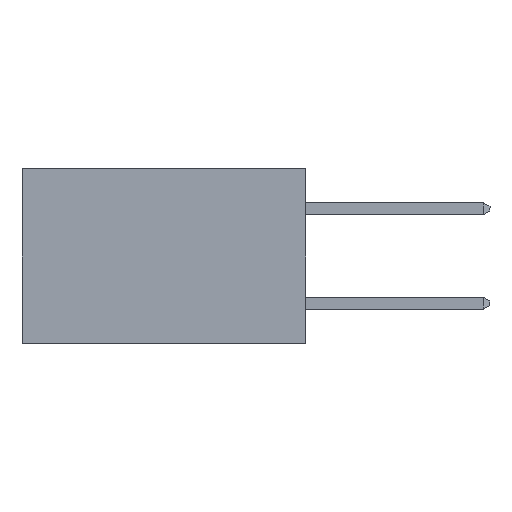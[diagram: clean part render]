
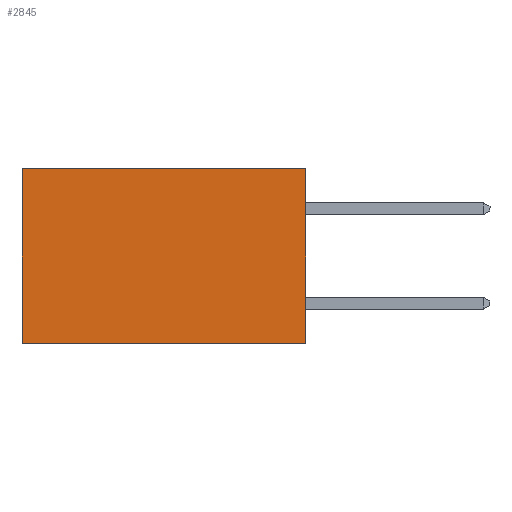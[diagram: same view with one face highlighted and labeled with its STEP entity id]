
A CAD part, left-side view. The second image highlights one B-rep face of the part: STEP entity #2845.
In plain terms, the highlighted planar face has unit normal (-1, 0, 0).
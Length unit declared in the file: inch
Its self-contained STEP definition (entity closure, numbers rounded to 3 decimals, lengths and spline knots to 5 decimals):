
#236 = EDGE_CURVE ( 'NONE', #4190, #8063, #8089, .T. ) ;
#643 = ORIENTED_EDGE ( 'NONE', *, *, #4900, .F. ) ;
#648 = VECTOR ( 'NONE', #2766, 39.37008 ) ;
#804 = VECTOR ( 'NONE', #7829, 39.37008 ) ;
#814 = CARTESIAN_POINT ( 'NONE',  ( 0.2615, 0.6, -0.37 ) ) ;
#836 = LINE ( 'NONE', #5321, #648 ) ;
#911 = LINE ( 'NONE', #2721, #804 ) ;
#1516 = FACE_OUTER_BOUND ( 'NONE', #3826, .T. ) ;
#1579 = AXIS2_PLACEMENT_3D ( 'NONE', #5293, #4053, #4133 ) ;
#1909 = VECTOR ( 'NONE', #5614, 39.37008 ) ;
#2027 = ORIENTED_EDGE ( 'NONE', *, *, #5653, .F. ) ;
#2721 = CARTESIAN_POINT ( 'NONE',  ( 0.2615, 0., -0.37 ) ) ;
#2766 = DIRECTION ( 'NONE',  ( 0., 1., 0. ) ) ;
#2781 = VECTOR ( 'NONE', #2974, 39.37008 ) ;
#2845 = ADVANCED_FACE ( 'NONE', ( #1516 ), #4671, .F. ) ;
#2974 = DIRECTION ( 'NONE',  ( 0., 0., -1. ) ) ;
#3267 = EDGE_CURVE ( 'NONE', #3334, #4190, #836, .T. ) ;
#3334 = VERTEX_POINT ( 'NONE', #3697 ) ;
#3697 = CARTESIAN_POINT ( 'NONE',  ( 0.2615, 0., 0. ) ) ;
#3826 = EDGE_LOOP ( 'NONE', ( #4795, #643, #2027, #5161 ) ) ;
#3866 = LINE ( 'NONE', #4975, #1909 ) ;
#4053 = DIRECTION ( 'NONE',  ( 1., 0., 0. ) ) ;
#4133 = DIRECTION ( 'NONE',  ( 0., 0., -1. ) ) ;
#4190 = VERTEX_POINT ( 'NONE', #6688 ) ;
#4671 = PLANE ( 'NONE',  #1579 ) ;
#4795 = ORIENTED_EDGE ( 'NONE', *, *, #236, .T. ) ;
#4900 = EDGE_CURVE ( 'NONE', #7779, #8063, #911, .T. ) ;
#4975 = CARTESIAN_POINT ( 'NONE',  ( 0.2615, 0., -0.37 ) ) ;
#5161 = ORIENTED_EDGE ( 'NONE', *, *, #3267, .T. ) ;
#5293 = CARTESIAN_POINT ( 'NONE',  ( 0.2615, 0., -0.37 ) ) ;
#5321 = CARTESIAN_POINT ( 'NONE',  ( 0.2615, 0., 0. ) ) ;
#5614 = DIRECTION ( 'NONE',  ( 0., 0., -1. ) ) ;
#5653 = EDGE_CURVE ( 'NONE', #3334, #7779, #3866, .T. ) ;
#6230 = CARTESIAN_POINT ( 'NONE',  ( 0.2615, 0.6, -0.37 ) ) ;
#6688 = CARTESIAN_POINT ( 'NONE',  ( 0.2615, 0.6, 0. ) ) ;
#6852 = CARTESIAN_POINT ( 'NONE',  ( 0.2615, 0., -0.37 ) ) ;
#7779 = VERTEX_POINT ( 'NONE', #6852 ) ;
#7829 = DIRECTION ( 'NONE',  ( 0., 1., 0. ) ) ;
#8063 = VERTEX_POINT ( 'NONE', #814 ) ;
#8089 = LINE ( 'NONE', #6230, #2781 ) ;
